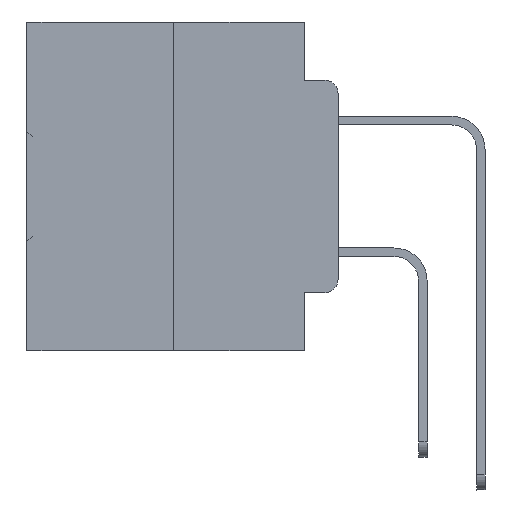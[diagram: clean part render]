
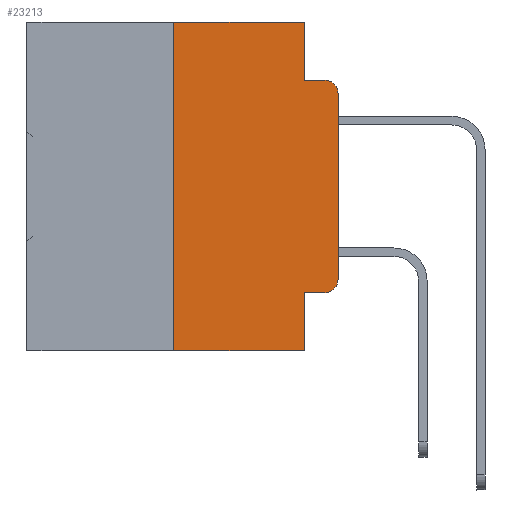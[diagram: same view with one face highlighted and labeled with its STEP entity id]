
A CAD part, left-side view. The second image highlights one B-rep face of the part: STEP entity #23213.
In plain terms, the highlighted planar face has unit normal (-1, 0, 0).
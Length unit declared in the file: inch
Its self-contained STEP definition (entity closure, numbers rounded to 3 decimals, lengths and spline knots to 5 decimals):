
#410 = DIRECTION ( 'NONE',  ( 0., 0., -1. ) ) ;
#546 = VECTOR ( 'NONE', #29434, 39.37008 ) ;
#1148 = VECTOR ( 'NONE', #16589, 39.37008 ) ;
#1789 = DIRECTION ( 'NONE',  ( 0., -1., 0. ) ) ;
#1909 = VERTEX_POINT ( 'NONE', #10663 ) ;
#2053 = DIRECTION ( 'NONE',  ( -1., 0., 0. ) ) ;
#3002 = DIRECTION ( 'NONE',  ( 0., 0., 1. ) ) ;
#3036 = DIRECTION ( 'NONE',  ( -1., 0., 0. ) ) ;
#3261 = FACE_OUTER_BOUND ( 'NONE', #27698, .T. ) ;
#3271 = VERTEX_POINT ( 'NONE', #21265 ) ;
#3286 = LINE ( 'NONE', #25495, #32339 ) ;
#3521 = CIRCLE ( 'NONE', #30876, 0.02 ) ;
#5095 = CARTESIAN_POINT ( 'NONE',  ( 0., 0.051, -0.4115 ) ) ;
#6743 = VECTOR ( 'NONE', #20473, 39.37008 ) ;
#6838 = EDGE_CURVE ( 'NONE', #22100, #25415, #8890, .T. ) ;
#7344 = ORIENTED_EDGE ( 'NONE', *, *, #22392, .T. ) ;
#7591 = ORIENTED_EDGE ( 'NONE', *, *, #35632, .F. ) ;
#7920 = CARTESIAN_POINT ( 'NONE',  ( 0., 0., -0.3915 ) ) ;
#7958 = CARTESIAN_POINT ( 'NONE',  ( 0., 0.473, 0. ) ) ;
#7979 = VECTOR ( 'NONE', #410, 39.37008 ) ;
#8001 = DIRECTION ( 'NONE',  ( 0., -1., 0. ) ) ;
#8313 = LINE ( 'NONE', #23827, #546 ) ;
#8470 = ORIENTED_EDGE ( 'NONE', *, *, #20303, .F. ) ;
#8517 = CARTESIAN_POINT ( 'NONE',  ( 0., 0.051, 0. ) ) ;
#8661 = VERTEX_POINT ( 'NONE', #34737 ) ;
#8890 = LINE ( 'NONE', #33653, #1148 ) ;
#9096 = CARTESIAN_POINT ( 'NONE',  ( 0., 0.051, 0. ) ) ;
#10663 = CARTESIAN_POINT ( 'NONE',  ( 0., 0.25, 0. ) ) ;
#10709 = EDGE_CURVE ( 'NONE', #25415, #17928, #30509, .T. ) ;
#10730 = VECTOR ( 'NONE', #27652, 39.37008 ) ;
#11813 = LINE ( 'NONE', #5095, #25791 ) ;
#12048 = ORIENTED_EDGE ( 'NONE', *, *, #6838, .F. ) ;
#12279 = CARTESIAN_POINT ( 'NONE',  ( 0., 0.051, -0.4115 ) ) ;
#12440 = CARTESIAN_POINT ( 'NONE',  ( 0., 0.25, -0.5 ) ) ;
#12481 = LINE ( 'NONE', #24815, #10730 ) ;
#12575 = EDGE_CURVE ( 'NONE', #34950, #17928, #32527, .T. ) ;
#13519 = AXIS2_PLACEMENT_3D ( 'NONE', #7958, #35883, #19254 ) ;
#13927 = VECTOR ( 'NONE', #1789, 39.37008 ) ;
#14462 = EDGE_CURVE ( 'NONE', #25553, #34950, #22581, .T. ) ;
#14638 = ORIENTED_EDGE ( 'NONE', *, *, #10709, .F. ) ;
#14909 = AXIS2_PLACEMENT_3D ( 'NONE', #19085, #2053, #21881 ) ;
#16261 = CARTESIAN_POINT ( 'NONE',  ( 0., 0.02, -0.0885 ) ) ;
#16309 = ORIENTED_EDGE ( 'NONE', *, *, #12575, .T. ) ;
#16438 = PLANE ( 'NONE',  #13519 ) ;
#16589 = DIRECTION ( 'NONE',  ( 0., 0., -1. ) ) ;
#16857 = CARTESIAN_POINT ( 'NONE',  ( 0., 0., -0.1085 ) ) ;
#17350 = ORIENTED_EDGE ( 'NONE', *, *, #26378, .T. ) ;
#17564 = ORIENTED_EDGE ( 'NONE', *, *, #14462, .T. ) ;
#17928 = VERTEX_POINT ( 'NONE', #16261 ) ;
#18626 = CARTESIAN_POINT ( 'NONE',  ( 0., 0.051, -0.0885 ) ) ;
#18843 = CARTESIAN_POINT ( 'NONE',  ( 0., 0.051, -0.0885 ) ) ;
#19085 = CARTESIAN_POINT ( 'NONE',  ( 0., 0.02, -0.1085 ) ) ;
#19254 = DIRECTION ( 'NONE',  ( 0., 0., -1. ) ) ;
#19983 = VERTEX_POINT ( 'NONE', #12279 ) ;
#20017 = CARTESIAN_POINT ( 'NONE',  ( 0., 0.02, -0.3915 ) ) ;
#20303 = EDGE_CURVE ( 'NONE', #1909, #22100, #12481, .T. ) ;
#20473 = DIRECTION ( 'NONE',  ( 0., 0., 1. ) ) ;
#21265 = CARTESIAN_POINT ( 'NONE',  ( 0., 0.051, -0.5 ) ) ;
#21881 = DIRECTION ( 'NONE',  ( 0., 0., -1. ) ) ;
#22100 = VERTEX_POINT ( 'NONE', #8517 ) ;
#22392 = EDGE_CURVE ( 'NONE', #28692, #3271, #8313, .T. ) ;
#22581 = LINE ( 'NONE', #33866, #6743 ) ;
#22821 = DIRECTION ( 'NONE',  ( 0., 0., -1. ) ) ;
#23213 = ADVANCED_FACE ( 'NONE', ( #3261 ), #16438, .F. ) ;
#23827 = CARTESIAN_POINT ( 'NONE',  ( 0., 0.473, -0.5 ) ) ;
#24293 = ORIENTED_EDGE ( 'NONE', *, *, #30102, .T. ) ;
#24815 = CARTESIAN_POINT ( 'NONE',  ( 0., 0.473, 0. ) ) ;
#25196 = ORIENTED_EDGE ( 'NONE', *, *, #33814, .F. ) ;
#25415 = VERTEX_POINT ( 'NONE', #18626 ) ;
#25495 = CARTESIAN_POINT ( 'NONE',  ( 0., 0.25, 0. ) ) ;
#25553 = VERTEX_POINT ( 'NONE', #7920 ) ;
#25791 = VECTOR ( 'NONE', #8001, 39.37008 ) ;
#26378 = EDGE_CURVE ( 'NONE', #8661, #25553, #3521, .T. ) ;
#27652 = DIRECTION ( 'NONE',  ( 0., -1., 0. ) ) ;
#27698 = EDGE_LOOP ( 'NONE', ( #17564, #16309, #14638, #12048, #8470, #7591, #7344, #25196, #24293, #17350 ) ) ;
#28692 = VERTEX_POINT ( 'NONE', #12440 ) ;
#29434 = DIRECTION ( 'NONE',  ( 0., -1., 0. ) ) ;
#30102 = EDGE_CURVE ( 'NONE', #19983, #8661, #11813, .T. ) ;
#30509 = LINE ( 'NONE', #18843, #13927 ) ;
#30876 = AXIS2_PLACEMENT_3D ( 'NONE', #20017, #3036, #22821 ) ;
#31195 = LINE ( 'NONE', #9096, #7979 ) ;
#32339 = VECTOR ( 'NONE', #3002, 39.37008 ) ;
#32527 = CIRCLE ( 'NONE', #14909, 0.02 ) ;
#33653 = CARTESIAN_POINT ( 'NONE',  ( 0., 0.051, 0. ) ) ;
#33814 = EDGE_CURVE ( 'NONE', #19983, #3271, #31195, .T. ) ;
#33866 = CARTESIAN_POINT ( 'NONE',  ( 0., 0., 0. ) ) ;
#34737 = CARTESIAN_POINT ( 'NONE',  ( 0., 0.02, -0.4115 ) ) ;
#34950 = VERTEX_POINT ( 'NONE', #16857 ) ;
#35632 = EDGE_CURVE ( 'NONE', #28692, #1909, #3286, .T. ) ;
#35883 = DIRECTION ( 'NONE',  ( 1., 0., 0. ) ) ;
